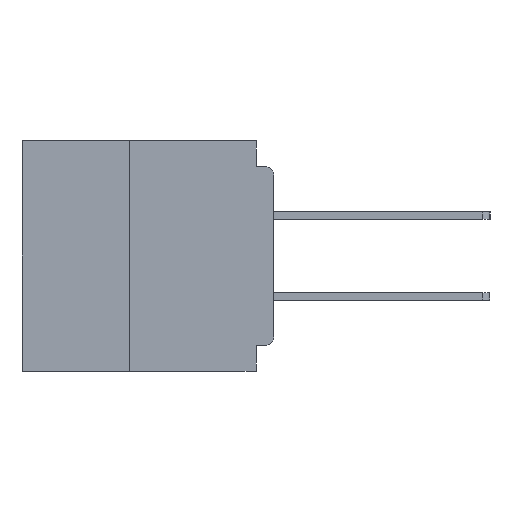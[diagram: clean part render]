
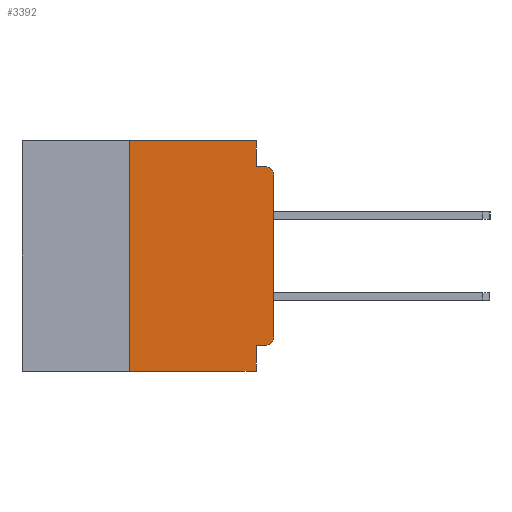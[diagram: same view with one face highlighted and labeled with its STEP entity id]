
A CAD part, left-side view. The second image highlights one B-rep face of the part: STEP entity #3392.
In plain terms, the highlighted planar face has unit normal (-1, 0, 0).
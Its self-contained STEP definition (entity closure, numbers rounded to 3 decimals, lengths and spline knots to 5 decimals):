
#384 = VERTEX_POINT ( 'NONE', #46234 ) ;
#626 = VERTEX_POINT ( 'NONE', #28614 ) ;
#680 = DIRECTION ( 'NONE',  ( 0., 0., -1. ) ) ;
#1058 = CARTESIAN_POINT ( 'NONE',  ( 0., 0.437, -0.4 ) ) ;
#3150 = VERTEX_POINT ( 'NONE', #3624 ) ;
#3392 = ADVANCED_FACE ( 'NONE', ( #4919 ), #30408, .F. ) ;
#3624 = CARTESIAN_POINT ( 'NONE',  ( 0., 0.015, -0.355 ) ) ;
#4438 = VERTEX_POINT ( 'NONE', #49261 ) ;
#4845 = ORIENTED_EDGE ( 'NONE', *, *, #12041, .T. ) ;
#4919 = FACE_OUTER_BOUND ( 'NONE', #62654, .T. ) ;
#5349 = LINE ( 'NONE', #28843, #32957 ) ;
#6085 = ORIENTED_EDGE ( 'NONE', *, *, #49725, .F. ) ;
#6461 = CARTESIAN_POINT ( 'NONE',  ( 0., 0.25, -0.4 ) ) ;
#7029 = DIRECTION ( 'NONE',  ( 0., 1., 0. ) ) ;
#8921 = EDGE_CURVE ( 'NONE', #41904, #26764, #19822, .T. ) ;
#10354 = VECTOR ( 'NONE', #51958, 39.37008 ) ;
#10522 = CARTESIAN_POINT ( 'NONE',  ( 0., 0., -0.045 ) ) ;
#11386 = CIRCLE ( 'NONE', #48341, 0.015 ) ;
#12041 = EDGE_CURVE ( 'NONE', #23076, #26764, #32433, .T. ) ;
#16451 = CARTESIAN_POINT ( 'NONE',  ( 0., 0.015, -0.06 ) ) ;
#16693 = DIRECTION ( 'NONE',  ( 0., -1., 0. ) ) ;
#17754 = CARTESIAN_POINT ( 'NONE',  ( 0., 0., -0.34 ) ) ;
#18407 = EDGE_CURVE ( 'NONE', #23076, #4438, #63279, .T. ) ;
#18668 = VECTOR ( 'NONE', #16693, 39.37008 ) ;
#19822 = LINE ( 'NONE', #24451, #50567 ) ;
#20896 = CIRCLE ( 'NONE', #51355, 0.015 ) ;
#21678 = DIRECTION ( 'NONE',  ( 0., 0., -1. ) ) ;
#23076 = VERTEX_POINT ( 'NONE', #6461 ) ;
#23132 = CARTESIAN_POINT ( 'NONE',  ( 0., 0.437, 0. ) ) ;
#23687 = VECTOR ( 'NONE', #29122, 39.37008 ) ;
#24440 = CARTESIAN_POINT ( 'NONE',  ( 0., 0., 0. ) ) ;
#24451 = CARTESIAN_POINT ( 'NONE',  ( 0., 0.031, -0.4 ) ) ;
#25119 = VERTEX_POINT ( 'NONE', #33745 ) ;
#26157 = VECTOR ( 'NONE', #48922, 39.37008 ) ;
#26764 = VERTEX_POINT ( 'NONE', #65543 ) ;
#27800 = ORIENTED_EDGE ( 'NONE', *, *, #45670, .F. ) ;
#28614 = CARTESIAN_POINT ( 'NONE',  ( 0., 0., -0.06 ) ) ;
#28843 = CARTESIAN_POINT ( 'NONE',  ( 0., 0.031, 0. ) ) ;
#29122 = DIRECTION ( 'NONE',  ( 0., 0., 1. ) ) ;
#30408 = PLANE ( 'NONE',  #31134 ) ;
#31134 = AXIS2_PLACEMENT_3D ( 'NONE', #56140, #66491, #35615 ) ;
#31712 = DIRECTION ( 'NONE',  ( -1., 0., 0. ) ) ;
#32433 = LINE ( 'NONE', #1058, #18668 ) ;
#32957 = VECTOR ( 'NONE', #64919, 39.37008 ) ;
#33399 = ORIENTED_EDGE ( 'NONE', *, *, #18407, .F. ) ;
#33745 = CARTESIAN_POINT ( 'NONE',  ( 0., 0.031, -0.045 ) ) ;
#33787 = LINE ( 'NONE', #53650, #35428 ) ;
#35368 = EDGE_CURVE ( 'NONE', #626, #61448, #20896, .T. ) ;
#35428 = VECTOR ( 'NONE', #7029, 39.37008 ) ;
#35615 = DIRECTION ( 'NONE',  ( 0., 0., -1. ) ) ;
#36780 = ORIENTED_EDGE ( 'NONE', *, *, #35368, .T. ) ;
#37469 = ORIENTED_EDGE ( 'NONE', *, *, #60658, .F. ) ;
#40495 = EDGE_CURVE ( 'NONE', #25119, #61448, #63782, .T. ) ;
#41904 = VERTEX_POINT ( 'NONE', #47375 ) ;
#42986 = VECTOR ( 'NONE', #50665, 39.37008 ) ;
#44505 = CARTESIAN_POINT ( 'NONE',  ( 0., 0.25, -0.4 ) ) ;
#45670 = EDGE_CURVE ( 'NONE', #4438, #384, #55266, .T. ) ;
#46234 = CARTESIAN_POINT ( 'NONE',  ( 0., 0.031, 0. ) ) ;
#47375 = CARTESIAN_POINT ( 'NONE',  ( 0., 0.031, -0.355 ) ) ;
#48311 = ORIENTED_EDGE ( 'NONE', *, *, #66935, .T. ) ;
#48341 = AXIS2_PLACEMENT_3D ( 'NONE', #62625, #31712, #680 ) ;
#48609 = ORIENTED_EDGE ( 'NONE', *, *, #40495, .F. ) ;
#48778 = CARTESIAN_POINT ( 'NONE',  ( 0., 0.015, -0.045 ) ) ;
#48922 = DIRECTION ( 'NONE',  ( 0., -1., 0. ) ) ;
#49261 = CARTESIAN_POINT ( 'NONE',  ( 0., 0.25, 0. ) ) ;
#49725 = EDGE_CURVE ( 'NONE', #3150, #41904, #33787, .T. ) ;
#50567 = VECTOR ( 'NONE', #55409, 39.37008 ) ;
#50665 = DIRECTION ( 'NONE',  ( 0., 0., 1. ) ) ;
#51355 = AXIS2_PLACEMENT_3D ( 'NONE', #16451, #52614, #21678 ) ;
#51958 = DIRECTION ( 'NONE',  ( 0., -1., 0. ) ) ;
#52614 = DIRECTION ( 'NONE',  ( -1., 0., 0. ) ) ;
#53029 = VERTEX_POINT ( 'NONE', #17754 ) ;
#53650 = CARTESIAN_POINT ( 'NONE',  ( 0., 0., -0.355 ) ) ;
#55266 = LINE ( 'NONE', #23132, #26157 ) ;
#55409 = DIRECTION ( 'NONE',  ( 0., 0., -1. ) ) ;
#56140 = CARTESIAN_POINT ( 'NONE',  ( 0., 0.437, 0. ) ) ;
#56677 = LINE ( 'NONE', #24440, #42986 ) ;
#58223 = EDGE_CURVE ( 'NONE', #3150, #53029, #11386, .T. ) ;
#60658 = EDGE_CURVE ( 'NONE', #384, #25119, #5349, .T. ) ;
#61448 = VERTEX_POINT ( 'NONE', #48778 ) ;
#62517 = ORIENTED_EDGE ( 'NONE', *, *, #58223, .T. ) ;
#62625 = CARTESIAN_POINT ( 'NONE',  ( 0., 0.015, -0.34 ) ) ;
#62654 = EDGE_LOOP ( 'NONE', ( #48311, #36780, #48609, #37469, #27800, #33399, #4845, #65433, #6085, #62517 ) ) ;
#63279 = LINE ( 'NONE', #44505, #23687 ) ;
#63782 = LINE ( 'NONE', #10522, #10354 ) ;
#64919 = DIRECTION ( 'NONE',  ( 0., 0., -1. ) ) ;
#65433 = ORIENTED_EDGE ( 'NONE', *, *, #8921, .F. ) ;
#65543 = CARTESIAN_POINT ( 'NONE',  ( 0., 0.031, -0.4 ) ) ;
#66491 = DIRECTION ( 'NONE',  ( 1., 0., 0. ) ) ;
#66935 = EDGE_CURVE ( 'NONE', #53029, #626, #56677, .T. ) ;
